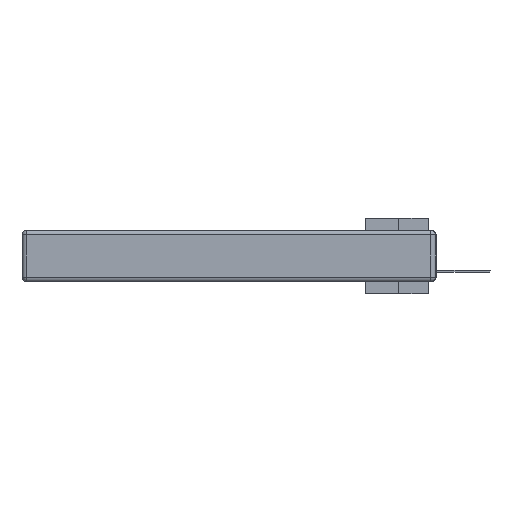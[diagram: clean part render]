
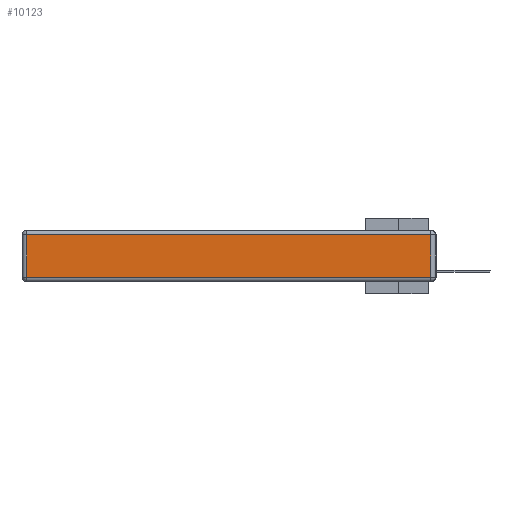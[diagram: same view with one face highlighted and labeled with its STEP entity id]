
A CAD part, left-side view. The second image highlights one B-rep face of the part: STEP entity #10123.
In plain terms, the highlighted planar face has unit normal (-1, 0, 0).
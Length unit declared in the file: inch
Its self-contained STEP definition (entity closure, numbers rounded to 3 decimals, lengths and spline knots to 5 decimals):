
#1326 = DIRECTION ( 'NONE',  ( 0., -1., 0. ) ) ;
#2362 = EDGE_CURVE ( 'NONE', #16900, #7318, #7837, .T. ) ;
#4389 = CARTESIAN_POINT ( 'NONE',  ( 0., 2.72, -0.313 ) ) ;
#5347 = DIRECTION ( 'NONE',  ( 0., 0., 1. ) ) ;
#6546 = LINE ( 'NONE', #31976, #8001 ) ;
#6736 = VERTEX_POINT ( 'NONE', #4389 ) ;
#7318 = VERTEX_POINT ( 'NONE', #26525 ) ;
#7837 = LINE ( 'NONE', #28107, #32278 ) ;
#8001 = VECTOR ( 'NONE', #9032, 39.37008 ) ;
#8303 = DIRECTION ( 'NONE',  ( 0., 0., 1. ) ) ;
#9032 = DIRECTION ( 'NONE',  ( 0., 0., -1. ) ) ;
#9458 = EDGE_CURVE ( 'NONE', #28647, #6736, #6546, .T. ) ;
#10123 = ADVANCED_FACE ( 'NONE', ( #23094 ), #28574, .T. ) ;
#13412 = DIRECTION ( 'NONE',  ( 0., 1., 0. ) ) ;
#14758 = CARTESIAN_POINT ( 'NONE',  ( 0., 2.72, -0.03 ) ) ;
#16074 = LINE ( 'NONE', #23231, #21966 ) ;
#16111 = DIRECTION ( 'NONE',  ( -1., 0., 0. ) ) ;
#16900 = VERTEX_POINT ( 'NONE', #22820 ) ;
#18954 = LINE ( 'NONE', #29089, #24673 ) ;
#21933 = ORIENTED_EDGE ( 'NONE', *, *, #27515, .T. ) ;
#21966 = VECTOR ( 'NONE', #13412, 39.37008 ) ;
#22820 = CARTESIAN_POINT ( 'NONE',  ( 0., 0.03, -0.313 ) ) ;
#23094 = FACE_OUTER_BOUND ( 'NONE', #28165, .T. ) ;
#23231 = CARTESIAN_POINT ( 'NONE',  ( 0., 2.75, -0.03 ) ) ;
#23377 = AXIS2_PLACEMENT_3D ( 'NONE', #25909, #16111, #8303 ) ;
#24673 = VECTOR ( 'NONE', #1326, 39.37008 ) ;
#25774 = ORIENTED_EDGE ( 'NONE', *, *, #32282, .T. ) ;
#25909 = CARTESIAN_POINT ( 'NONE',  ( 0., 0., -0.343 ) ) ;
#26525 = CARTESIAN_POINT ( 'NONE',  ( 0., 0.03, -0.03 ) ) ;
#27515 = EDGE_CURVE ( 'NONE', #7318, #28647, #16074, .T. ) ;
#28107 = CARTESIAN_POINT ( 'NONE',  ( 0., 0.03, -0.343 ) ) ;
#28165 = EDGE_LOOP ( 'NONE', ( #25774, #28943, #21933, #32000 ) ) ;
#28574 = PLANE ( 'NONE',  #23377 ) ;
#28647 = VERTEX_POINT ( 'NONE', #14758 ) ;
#28943 = ORIENTED_EDGE ( 'NONE', *, *, #2362, .T. ) ;
#29089 = CARTESIAN_POINT ( 'NONE',  ( 0., 0., -0.313 ) ) ;
#31976 = CARTESIAN_POINT ( 'NONE',  ( 0., 2.72, -0.343 ) ) ;
#32000 = ORIENTED_EDGE ( 'NONE', *, *, #9458, .T. ) ;
#32278 = VECTOR ( 'NONE', #5347, 39.37008 ) ;
#32282 = EDGE_CURVE ( 'NONE', #6736, #16900, #18954, .T. ) ;
